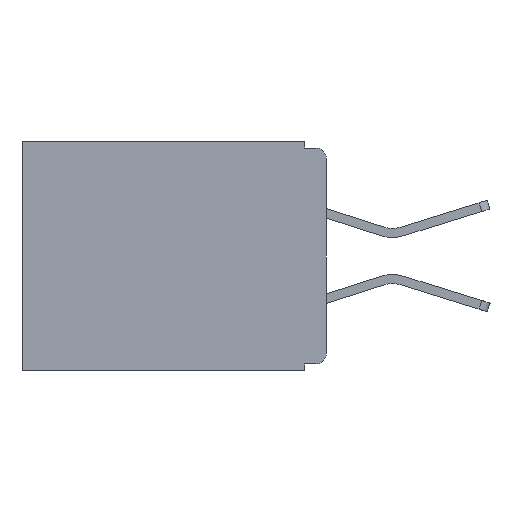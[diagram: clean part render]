
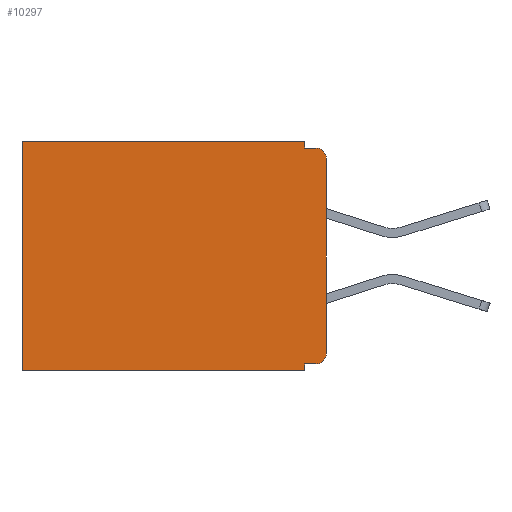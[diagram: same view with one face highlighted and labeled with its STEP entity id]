
A CAD part, left-side view. The second image highlights one B-rep face of the part: STEP entity #10297.
In plain terms, the highlighted planar face has unit normal (-1, 0, 0).
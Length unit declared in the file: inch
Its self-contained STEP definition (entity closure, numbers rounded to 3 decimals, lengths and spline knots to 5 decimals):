
#23 = ORIENTED_EDGE ( 'NONE', *, *, #2667, .F. ) ;
#30 = DIRECTION ( 'NONE',  ( 0., -1., 0. ) ) ;
#196 = EDGE_CURVE ( 'NONE', #10733, #2485, #9720, .T. ) ;
#815 = ORIENTED_EDGE ( 'NONE', *, *, #6328, .T. ) ;
#1316 = VERTEX_POINT ( 'NONE', #2981 ) ;
#1456 = PLANE ( 'NONE',  #10255 ) ;
#1969 = DIRECTION ( 'NONE',  ( 0., 1., 0. ) ) ;
#2167 = ORIENTED_EDGE ( 'NONE', *, *, #7632, .T. ) ;
#2170 = VECTOR ( 'NONE', #5951, 39.37008 ) ;
#2381 = VECTOR ( 'NONE', #30, 39.37008 ) ;
#2485 = VERTEX_POINT ( 'NONE', #4863 ) ;
#2526 = DIRECTION ( 'NONE',  ( 1., 0., 0. ) ) ;
#2667 = EDGE_CURVE ( 'NONE', #2485, #1316, #2700, .T. ) ;
#2677 = CARTESIAN_POINT ( 'NONE',  ( 0.3, 0.015, -0.025 ) ) ;
#2678 = DIRECTION ( 'NONE',  ( 0., 1., 0. ) ) ;
#2700 = LINE ( 'NONE', #12946, #2381 ) ;
#2739 = DIRECTION ( 'NONE',  ( 0., 1., 0. ) ) ;
#2966 = VECTOR ( 'NONE', #2739, 39.37008 ) ;
#2980 = VECTOR ( 'NONE', #1969, 39.37008 ) ;
#2981 = CARTESIAN_POINT ( 'NONE',  ( 0.3, 0.015, -0.01 ) ) ;
#3203 = CARTESIAN_POINT ( 'NONE',  ( 0.3, 0.031, -0.32 ) ) ;
#3241 = CARTESIAN_POINT ( 'NONE',  ( 0.3, 0., -0.33 ) ) ;
#3277 = VERTEX_POINT ( 'NONE', #3533 ) ;
#3533 = CARTESIAN_POINT ( 'NONE',  ( 0.3, 0.437, -0.33 ) ) ;
#3717 = CARTESIAN_POINT ( 'NONE',  ( 0.3, 0., -0.32 ) ) ;
#3752 = DIRECTION ( 'NONE',  ( 0., 0., -1. ) ) ;
#3895 = CARTESIAN_POINT ( 'NONE',  ( 0.3, 0.437, 0. ) ) ;
#4086 = CIRCLE ( 'NONE', #8992, 0.015 ) ;
#4242 = VERTEX_POINT ( 'NONE', #3895 ) ;
#4443 = LINE ( 'NONE', #11077, #11636 ) ;
#4472 = CARTESIAN_POINT ( 'NONE',  ( 0.3, 0.015, -0.305 ) ) ;
#4863 = CARTESIAN_POINT ( 'NONE',  ( 0.3, 0.031, -0.01 ) ) ;
#4904 = LINE ( 'NONE', #12809, #2170 ) ;
#5153 = VECTOR ( 'NONE', #7503, 39.37008 ) ;
#5212 = ORIENTED_EDGE ( 'NONE', *, *, #196, .F. ) ;
#5492 = DIRECTION ( 'NONE',  ( 0., 0., -1. ) ) ;
#5670 = ORIENTED_EDGE ( 'NONE', *, *, #7064, .F. ) ;
#5810 = VERTEX_POINT ( 'NONE', #7204 ) ;
#5951 = DIRECTION ( 'NONE',  ( 0., 0., -1. ) ) ;
#5959 = LINE ( 'NONE', #8706, #2966 ) ;
#5965 = ORIENTED_EDGE ( 'NONE', *, *, #11200, .F. ) ;
#5970 = LINE ( 'NONE', #7032, #2980 ) ;
#6012 = EDGE_CURVE ( 'NONE', #4242, #3277, #4904, .T. ) ;
#6239 = DIRECTION ( 'NONE',  ( 0., 0., -1. ) ) ;
#6328 = EDGE_CURVE ( 'NONE', #5810, #7129, #9016, .T. ) ;
#6597 = EDGE_LOOP ( 'NONE', ( #7527, #2167, #23, #5212, #10698, #10830, #5670, #5965, #8855, #815 ) ) ;
#6605 = EDGE_CURVE ( 'NONE', #10733, #4242, #5970, .T. ) ;
#6743 = EDGE_CURVE ( 'NONE', #10726, #7129, #12245, .T. ) ;
#7032 = CARTESIAN_POINT ( 'NONE',  ( 0.3, 0., 0. ) ) ;
#7064 = EDGE_CURVE ( 'NONE', #9031, #3277, #5959, .T. ) ;
#7129 = VERTEX_POINT ( 'NONE', #10691 ) ;
#7204 = CARTESIAN_POINT ( 'NONE',  ( 0.3, 0.015, -0.32 ) ) ;
#7405 = FACE_OUTER_BOUND ( 'NONE', #6597, .T. ) ;
#7503 = DIRECTION ( 'NONE',  ( 0., 0., -1. ) ) ;
#7527 = ORIENTED_EDGE ( 'NONE', *, *, #6743, .F. ) ;
#7632 = EDGE_CURVE ( 'NONE', #10726, #1316, #4086, .T. ) ;
#8161 = DIRECTION ( 'NONE',  ( 0., 0., -1. ) ) ;
#8389 = CARTESIAN_POINT ( 'NONE',  ( 0.3, 0.031, 0. ) ) ;
#8518 = CARTESIAN_POINT ( 'NONE',  ( 0.3, 0., -0.33 ) ) ;
#8706 = CARTESIAN_POINT ( 'NONE',  ( 0.3, 0., -0.33 ) ) ;
#8855 = ORIENTED_EDGE ( 'NONE', *, *, #11545, .F. ) ;
#8992 = AXIS2_PLACEMENT_3D ( 'NONE', #2677, #9605, #3752 ) ;
#9016 = CIRCLE ( 'NONE', #11532, 0.015 ) ;
#9031 = VERTEX_POINT ( 'NONE', #9539 ) ;
#9314 = VECTOR ( 'NONE', #8161, 39.37008 ) ;
#9467 = DIRECTION ( 'NONE',  ( 0., 0., -1. ) ) ;
#9539 = CARTESIAN_POINT ( 'NONE',  ( 0.3, 0.031, -0.33 ) ) ;
#9605 = DIRECTION ( 'NONE',  ( -1., 0., 0. ) ) ;
#9720 = LINE ( 'NONE', #10205, #5153 ) ;
#10205 = CARTESIAN_POINT ( 'NONE',  ( 0.3, 0.031, 0. ) ) ;
#10255 = AXIS2_PLACEMENT_3D ( 'NONE', #8518, #2526, #9467 ) ;
#10297 = ADVANCED_FACE ( 'NONE', ( #7405 ), #1456, .F. ) ;
#10691 = CARTESIAN_POINT ( 'NONE',  ( 0.3, 0., -0.305 ) ) ;
#10698 = ORIENTED_EDGE ( 'NONE', *, *, #6605, .T. ) ;
#10726 = VERTEX_POINT ( 'NONE', #12276 ) ;
#10733 = VERTEX_POINT ( 'NONE', #8389 ) ;
#10830 = ORIENTED_EDGE ( 'NONE', *, *, #6012, .T. ) ;
#10851 = LINE ( 'NONE', #3717, #11159 ) ;
#11077 = CARTESIAN_POINT ( 'NONE',  ( 0.3, 0.031, -0.33 ) ) ;
#11159 = VECTOR ( 'NONE', #2678, 39.37008 ) ;
#11200 = EDGE_CURVE ( 'NONE', #12724, #9031, #4443, .T. ) ;
#11322 = DIRECTION ( 'NONE',  ( -1., 0., 0. ) ) ;
#11532 = AXIS2_PLACEMENT_3D ( 'NONE', #4472, #11322, #5492 ) ;
#11545 = EDGE_CURVE ( 'NONE', #5810, #12724, #10851, .T. ) ;
#11636 = VECTOR ( 'NONE', #6239, 39.37008 ) ;
#12245 = LINE ( 'NONE', #3241, #9314 ) ;
#12276 = CARTESIAN_POINT ( 'NONE',  ( 0.3, 0., -0.025 ) ) ;
#12724 = VERTEX_POINT ( 'NONE', #3203 ) ;
#12809 = CARTESIAN_POINT ( 'NONE',  ( 0.3, 0.437, -0.33 ) ) ;
#12946 = CARTESIAN_POINT ( 'NONE',  ( 0.3, 0., -0.01 ) ) ;
